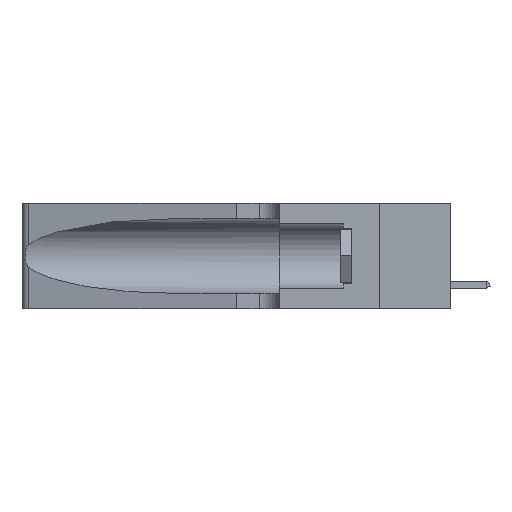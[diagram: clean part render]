
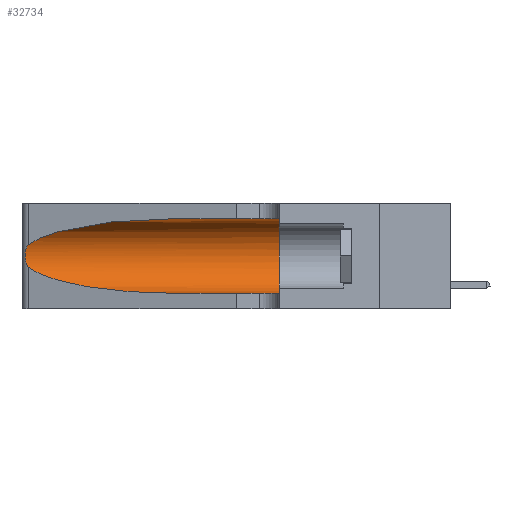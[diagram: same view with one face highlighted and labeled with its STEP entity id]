
A CAD part, left-side view. The second image highlights one B-rep face of the part: STEP entity #32734.
In plain terms, the highlighted cylindrical face has radius 3.308 mm (diameter 6.617 mm), a partial arc.
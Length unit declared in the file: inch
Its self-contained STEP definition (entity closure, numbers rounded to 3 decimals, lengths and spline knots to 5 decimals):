
#1275 = CARTESIAN_POINT ( 'NONE',  ( 0.25787, 1.23484, 0.2124 ) ) ;
#1376 = EDGE_CURVE ( 'NONE', #26506, #13152, #12367, .T. ) ;
#2907 = AXIS2_PLACEMENT_3D ( 'NONE', #22239, #37793, #34476 ) ;
#3866 = LINE ( 'NONE', #27792, #5900 ) ;
#5900 = VECTOR ( 'NONE', #28748, 39.37008 ) ;
#5983 = VERTEX_POINT ( 'NONE', #25671 ) ;
#6299 = CARTESIAN_POINT ( 'NONE',  ( 0.25487, 1.22718, 0.14631 ) ) ;
#6441 = CARTESIAN_POINT ( 'NONE',  ( 0.1305, 0.35, 0.185 ) ) ;
#6880 = VERTEX_POINT ( 'NONE', #10805 ) ;
#8124 = CARTESIAN_POINT ( 'NONE',  ( 0.1305, 0.72297, 0.31525 ) ) ;
#8338 = CARTESIAN_POINT ( 'NONE',  ( 0.1305, 0.72297, 0.05475 ) ) ;
#8476 = ORIENTED_EDGE ( 'NONE', *, *, #8563, .T. ) ;
#8563 = EDGE_CURVE ( 'NONE', #5983, #15078, #38300, .T. ) ;
#10184 = EDGE_CURVE ( 'NONE', #31402, #6880, #24175, .T. ) ;
#10805 = CARTESIAN_POINT ( 'NONE',  ( 0.25487, 1.22718, 0.22369 ) ) ;
#11255 = CARTESIAN_POINT ( 'NONE',  ( 0.26018, 1.23835, 0.19895 ) ) ;
#12367 = CIRCLE ( 'NONE', #19265, 0.13025 ) ;
#12695 = CARTESIAN_POINT ( 'NONE',  ( 0.25789, 1.23486, 0.15765 ) ) ;
#12785 = CARTESIAN_POINT ( 'NONE',  ( 0.25487, 1.22718, 0.22369 ) ) ;
#12820 = ORIENTED_EDGE ( 'NONE', *, *, #15983, .T. ) ;
#12993 = CARTESIAN_POINT ( 'NONE',  ( 0.1305, 0.35, 0.31525 ) ) ;
#13152 = VERTEX_POINT ( 'NONE', #30992 ) ;
#13889 = CARTESIAN_POINT ( 'NONE',  ( 0.18966, 0.96281, 0.05475 ) ) ;
#14037 = CARTESIAN_POINT ( 'NONE',  ( 0.1305, 0.72297, 0.05475 ) ) ;
#14244 = B_SPLINE_CURVE_WITH_KNOTS ( 'NONE', 3,
 ( #12785, #18153, #31157, #1275, #32237, #11255, #37688, #24390, #26831, #36702, #12695, #28207, #24192, #6299 ),
 .UNSPECIFIED., .F., .F.,
 ( 4, 2, 2, 2, 2, 2, 4 ),
 ( 0., 0.00027, 0.00053, 0.00107, 0.0016, 0.00187, 0.00214 ),
 .UNSPECIFIED. ) ;
#15078 = VERTEX_POINT ( 'NONE', #8338 ) ;
#15554 = DIRECTION ( 'NONE',  ( 0., 0., 1. ) ) ;
#15983 = EDGE_CURVE ( 'NONE', #6880, #5983, #14244, .T. ) ;
#16827 = CARTESIAN_POINT ( 'NONE',  ( 0.1305, 1.61858, 0.05475 ) ) ;
#16951 = ORIENTED_EDGE ( 'NONE', *, *, #10184, .T. ) ;
#17087 = CARTESIAN_POINT ( 'NONE',  ( 0.25487, 1.22718, 0.14631 ) ) ;
#18153 = CARTESIAN_POINT ( 'NONE',  ( 0.25555, 1.22994, 0.2215 ) ) ;
#19001 = CARTESIAN_POINT ( 'NONE',  ( 0.18966, 0.96281, 0.31525 ) ) ;
#19265 = AXIS2_PLACEMENT_3D ( 'NONE', #6441, #27489, #15554 ) ;
#19734 = ORIENTED_EDGE ( 'NONE', *, *, #33742, .F. ) ;
#21303 = EDGE_CURVE ( 'NONE', #15078, #13152, #28875, .T. ) ;
#22239 = CARTESIAN_POINT ( 'NONE',  ( 0.1305, 1.61858, 0.185 ) ) ;
#22430 = CARTESIAN_POINT ( 'NONE',  ( 0.2373, 1.15595, 0.28018 ) ) ;
#22700 = ORIENTED_EDGE ( 'NONE', *, *, #21303, .T. ) ;
#23181 = CARTESIAN_POINT ( 'NONE',  ( 0.2373, 1.15595, 0.08982 ) ) ;
#24175 =( BOUNDED_CURVE ( )  B_SPLINE_CURVE ( 3, ( #8124, #19001, #22430, #27810 ),
 .UNSPECIFIED., .F., .F. ) 
 B_SPLINE_CURVE_WITH_KNOTS ( ( 4, 4 ),
 ( 1.5708, 2.84003 ),
 .UNSPECIFIED. ) 
 CURVE ( )  GEOMETRIC_REPRESENTATION_ITEM ( )  RATIONAL_B_SPLINE_CURVE ( ( 1., 0.87, 0.87, 1. ) ) 
 REPRESENTATION_ITEM ( '' )  );
#24192 = CARTESIAN_POINT ( 'NONE',  ( 0.25555, 1.22993, 0.14849 ) ) ;
#24390 = CARTESIAN_POINT ( 'NONE',  ( 0.26075, 1.23896, 0.178 ) ) ;
#25671 = CARTESIAN_POINT ( 'NONE',  ( 0.25487, 1.22718, 0.14631 ) ) ;
#26506 = VERTEX_POINT ( 'NONE', #12993 ) ;
#26824 = FACE_OUTER_BOUND ( 'NONE', #34236, .T. ) ;
#26831 = CARTESIAN_POINT ( 'NONE',  ( 0.26017, 1.23833, 0.17102 ) ) ;
#27489 = DIRECTION ( 'NONE',  ( 0., 1., 0. ) ) ;
#27792 = CARTESIAN_POINT ( 'NONE',  ( 0.1305, 1.61858, 0.31525 ) ) ;
#27810 = CARTESIAN_POINT ( 'NONE',  ( 0.25487, 1.22718, 0.22369 ) ) ;
#28207 = CARTESIAN_POINT ( 'NONE',  ( 0.25639, 1.23186, 0.15144 ) ) ;
#28748 = DIRECTION ( 'NONE',  ( 0., -1., 0. ) ) ;
#28875 = LINE ( 'NONE', #16827, #38899 ) ;
#29558 = ORIENTED_EDGE ( 'NONE', *, *, #1376, .F. ) ;
#30992 = CARTESIAN_POINT ( 'NONE',  ( 0.1305, 0.35, 0.05475 ) ) ;
#31157 = CARTESIAN_POINT ( 'NONE',  ( 0.25639, 1.23184, 0.21858 ) ) ;
#31402 = VERTEX_POINT ( 'NONE', #32949 ) ;
#32237 = CARTESIAN_POINT ( 'NONE',  ( 0.25854, 1.2359, 0.20912 ) ) ;
#32734 = ADVANCED_FACE ( 'NONE', ( #26824 ), #33869, .F. ) ;
#32949 = CARTESIAN_POINT ( 'NONE',  ( 0.1305, 0.72297, 0.31525 ) ) ;
#33742 = EDGE_CURVE ( 'NONE', #31402, #26506, #3866, .T. ) ;
#33869 = CYLINDRICAL_SURFACE ( 'NONE', #2907, 0.13025 ) ;
#34236 = EDGE_LOOP ( 'NONE', ( #16951, #12820, #8476, #22700, #29558, #19734 ) ) ;
#34476 = DIRECTION ( 'NONE',  ( 0., 0., -1. ) ) ;
#35941 = DIRECTION ( 'NONE',  ( 0., -1., 0. ) ) ;
#36702 = CARTESIAN_POINT ( 'NONE',  ( 0.25856, 1.23593, 0.16098 ) ) ;
#37688 = CARTESIAN_POINT ( 'NONE',  ( 0.26075, 1.23896, 0.19203 ) ) ;
#37793 = DIRECTION ( 'NONE',  ( 0., -1., 0. ) ) ;
#38300 =( BOUNDED_CURVE ( )  B_SPLINE_CURVE ( 3, ( #17087, #23181, #13889, #14037 ),
 .UNSPECIFIED., .F., .T. ) 
 B_SPLINE_CURVE_WITH_KNOTS ( ( 4, 4 ),
 ( 3.44316, 4.71239 ),
 .UNSPECIFIED. ) 
 CURVE ( )  GEOMETRIC_REPRESENTATION_ITEM ( )  RATIONAL_B_SPLINE_CURVE ( ( 1., 0.87, 0.87, 1. ) ) 
 REPRESENTATION_ITEM ( '' )  );
#38899 = VECTOR ( 'NONE', #35941, 39.37008 ) ;
